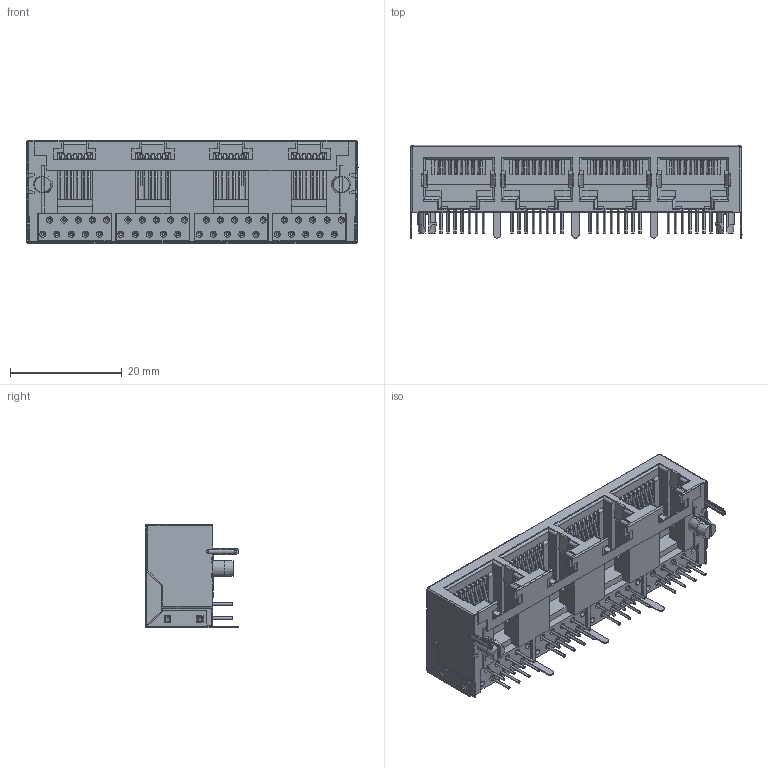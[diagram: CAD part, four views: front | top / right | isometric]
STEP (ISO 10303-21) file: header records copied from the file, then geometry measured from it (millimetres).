
FILE_DESCRIPTION (( 'STEP AP203' ), '1' );
FILE_NAME ('RJ60048862N00101.STEP', '2020-01-15T19:53:46', ( '' ), ( '' ), 'SwSTEP 2.0', 'SolidWorks 2016', '' );
FILE_SCHEMA (( 'CONFIG_CONTROL_DESIGN' ));
Length unit declared in the file: millimetre
Products named in the file (4): RJ60048862N00101; 60 Contacts_8P8C; 60 Insulator; 60 Shield
Assembly tree (6 placements, depth 2):
  RJ60048862N00101
    60 Insulator
    60 Shield
    60 Contacts_8P8C  x4
Bounding box: 59.3 x 16.65 x 18.4 mm (x, y, z)
Volume: 7013.3 mm3; surface area: 18560.1 mm2
Topology: 34 solids, 34 shells, 2562 faces, 7261 edges, 4735 vertices
Faces by surface type: plane 1489, cylinder 715, torus 192, cone 124, bspline 42
Entity records: 76204 total; most frequent: CARTESIAN_POINT 16502, ORIENTED_EDGE 12890, DIRECTION 11811, EDGE_CURVE 6445, LINE 4829, VECTOR 4829, VERTEX_POINT 4207, AXIS2_PLACEMENT_3D 3491
